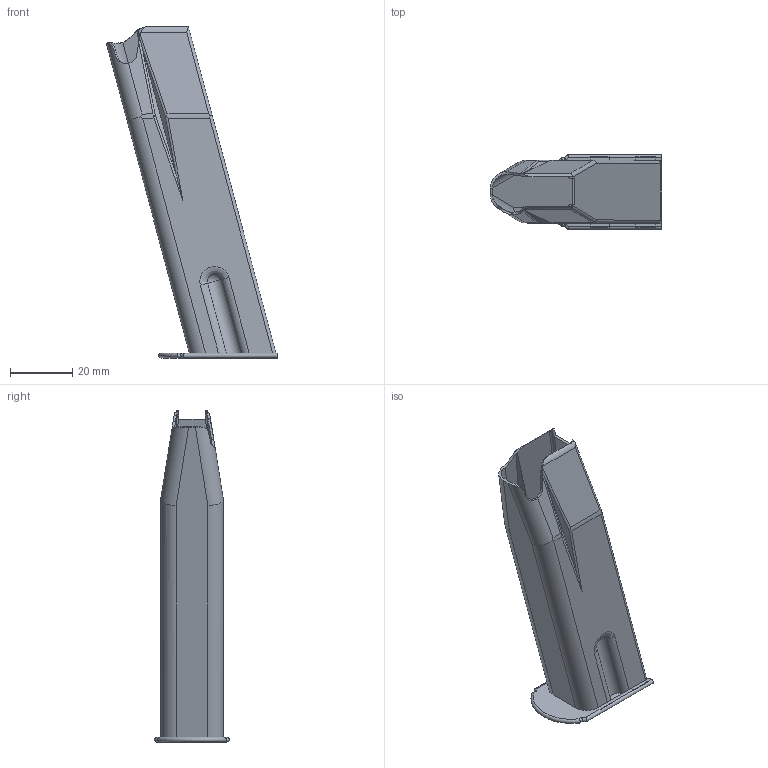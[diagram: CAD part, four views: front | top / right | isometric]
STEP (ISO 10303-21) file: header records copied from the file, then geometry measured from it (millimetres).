
FILE_DESCRIPTION(/* description */ ('baseBody_CZ82'),/* implementation_level */ '2;1');
FILE_NAME(/* name */ 'CZ82_baseMagazine',/* time_stamp */ '2023-09-18T17:37:42-04:00',/* author */ ('George'),/* organization */ ('Archive 663'),/* preprocessor_version */ 'ST-DEVELOPER v16.7',/* originating_system */ 'Solid Edge',/* authorisation */ 'Unknown');
FILE_SCHEMA (('AUTOMOTIVE_DESIGN {1 0 10303 214 3 1 1}'));
Length unit declared in the file: millimetre
Products named in the file (3): CZ82_baseBody; CZ82_baseMagazinePlate; CZ82_baseMagazine
Assembly tree (2 placements, depth 2):
  CZ82_baseBody
    CZ82_baseMagazinePlate
    CZ82_baseMagazine
Bounding box: 55.1 x 24 x 106.75 mm (x, y, z)
Volume: 7632.5 mm3; surface area: 20606.2 mm2
Topology: 2 solids, 2 shells, 149 faces, 431 edges, 277 vertices
Faces by surface type: plane 66, cylinder 58, bspline 12, torus 9, sphere 4
Full cylindrical faces by diameter (mm): 6 x1
Entity records: 5028 total; most frequent: CARTESIAN_POINT 1140, ORIENTED_EDGE 834, DIRECTION 770, EDGE_CURVE 417, VERTEX_POINT 272, AXIS2_PLACEMENT_3D 266, LINE 238, VECTOR 238
